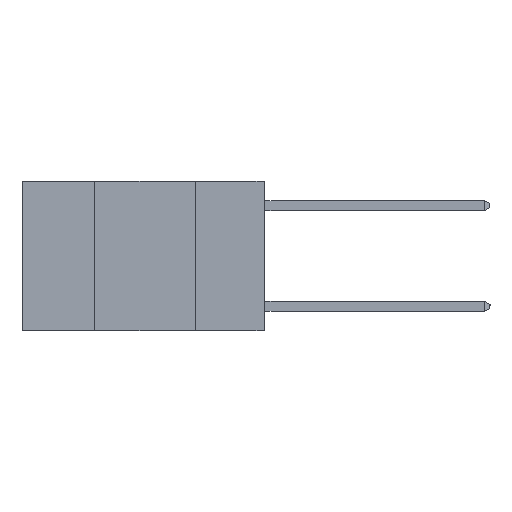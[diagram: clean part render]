
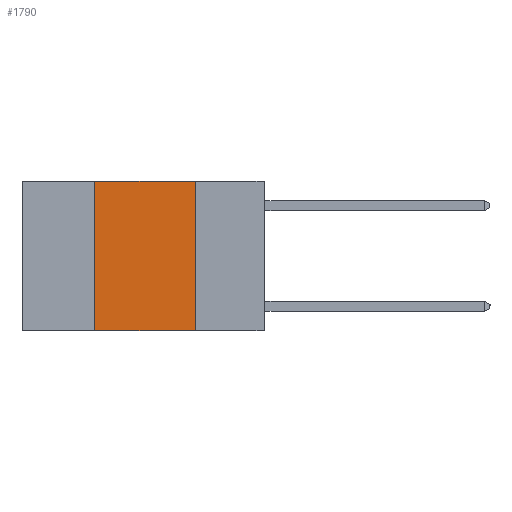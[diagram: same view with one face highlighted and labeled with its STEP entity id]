
A CAD part, left-side view. The second image highlights one B-rep face of the part: STEP entity #1790.
In plain terms, the highlighted planar face has unit normal (-1, 0, 0).
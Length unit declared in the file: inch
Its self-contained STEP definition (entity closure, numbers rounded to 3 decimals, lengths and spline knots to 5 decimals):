
#86 = CARTESIAN_POINT ( 'NONE',  ( 0., 0.17, -0.37 ) ) ;
#257 = CARTESIAN_POINT ( 'NONE',  ( 0., 0.42, 0. ) ) ;
#973 = ORIENTED_EDGE ( 'NONE', *, *, #1663, .F. ) ;
#1083 = ORIENTED_EDGE ( 'NONE', *, *, #5607, .F. ) ;
#1285 = DIRECTION ( 'NONE',  ( 0., 0., 1. ) ) ;
#1663 = EDGE_CURVE ( 'NONE', #12269, #4733, #9800, .T. ) ;
#1737 = VECTOR ( 'NONE', #8366, 39.37008 ) ;
#1790 = ADVANCED_FACE ( 'NONE', ( #8097 ), #5907, .F. ) ;
#2034 = EDGE_CURVE ( 'NONE', #10019, #12269, #12176, .T. ) ;
#2664 = CARTESIAN_POINT ( 'NONE',  ( 0., 0.6, 0. ) ) ;
#2723 = ORIENTED_EDGE ( 'NONE', *, *, #2034, .F. ) ;
#2830 = CARTESIAN_POINT ( 'NONE',  ( 0., 0.42, -0.37 ) ) ;
#2886 = CARTESIAN_POINT ( 'NONE',  ( 0., 0.6, 0. ) ) ;
#3901 = DIRECTION ( 'NONE',  ( 1., 0., 0. ) ) ;
#3983 = ORIENTED_EDGE ( 'NONE', *, *, #8140, .T. ) ;
#4568 = EDGE_LOOP ( 'NONE', ( #1083, #973, #2723, #3983 ) ) ;
#4691 = DIRECTION ( 'NONE',  ( 0., -1., 0. ) ) ;
#4727 = CARTESIAN_POINT ( 'NONE',  ( 0., 0.17, 0. ) ) ;
#4733 = VERTEX_POINT ( 'NONE', #6382 ) ;
#4813 = VECTOR ( 'NONE', #1285, 39.37008 ) ;
#5607 = EDGE_CURVE ( 'NONE', #4733, #7829, #9712, .T. ) ;
#5907 = PLANE ( 'NONE',  #6143 ) ;
#6023 = CARTESIAN_POINT ( 'NONE',  ( 0., 0.42, 0. ) ) ;
#6143 = AXIS2_PLACEMENT_3D ( 'NONE', #2886, #3901, #10545 ) ;
#6382 = CARTESIAN_POINT ( 'NONE',  ( 0., 0.17, 0. ) ) ;
#6578 = CARTESIAN_POINT ( 'NONE',  ( 0., 0.6, -0.37 ) ) ;
#7829 = VERTEX_POINT ( 'NONE', #86 ) ;
#8097 = FACE_OUTER_BOUND ( 'NONE', #4568, .T. ) ;
#8140 = EDGE_CURVE ( 'NONE', #10019, #7829, #9491, .T. ) ;
#8366 = DIRECTION ( 'NONE',  ( 0., -1., 0. ) ) ;
#9491 = LINE ( 'NONE', #6578, #1737 ) ;
#9712 = LINE ( 'NONE', #4727, #12363 ) ;
#9800 = LINE ( 'NONE', #2664, #12187 ) ;
#10019 = VERTEX_POINT ( 'NONE', #2830 ) ;
#10379 = DIRECTION ( 'NONE',  ( 0., 0., -1. ) ) ;
#10545 = DIRECTION ( 'NONE',  ( 0., 0., -1. ) ) ;
#12176 = LINE ( 'NONE', #257, #4813 ) ;
#12187 = VECTOR ( 'NONE', #4691, 39.37008 ) ;
#12269 = VERTEX_POINT ( 'NONE', #6023 ) ;
#12363 = VECTOR ( 'NONE', #10379, 39.37008 ) ;
